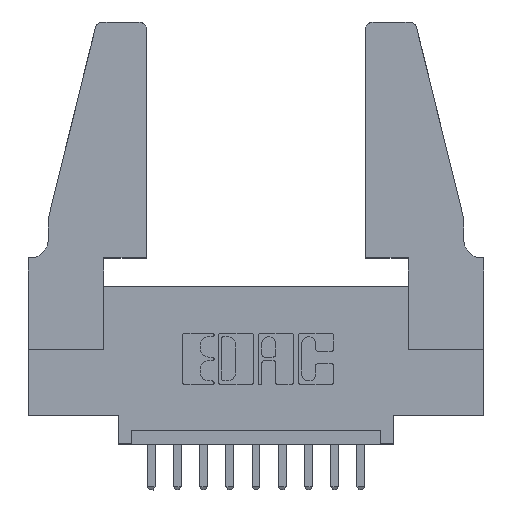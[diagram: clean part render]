
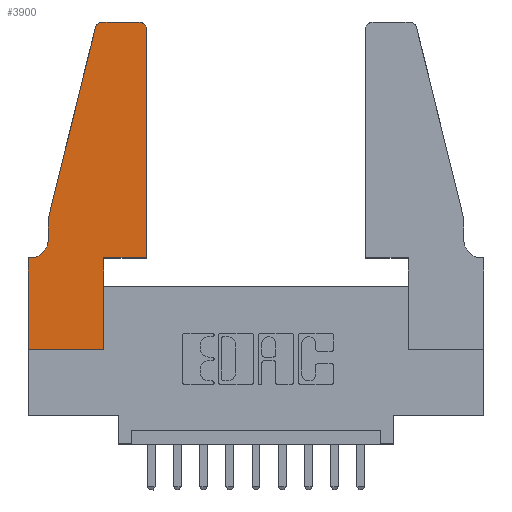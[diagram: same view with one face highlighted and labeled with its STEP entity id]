
A CAD part, top view. The second image highlights one B-rep face of the part: STEP entity #3900.
In plain terms, the highlighted planar face has unit normal (0, 0, 1).
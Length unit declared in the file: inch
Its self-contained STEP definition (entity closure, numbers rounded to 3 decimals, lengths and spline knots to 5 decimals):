
#124 = DIRECTION ( 'NONE',  ( 1., 0., 0. ) ) ;
#148 = DIRECTION ( 'NONE',  ( 1., 0., 0. ) ) ;
#385 = EDGE_CURVE ( 'NONE', #1958, #7361, #8464, .T. ) ;
#652 = ORIENTED_EDGE ( 'NONE', *, *, #8223, .T. ) ;
#665 = ORIENTED_EDGE ( 'NONE', *, *, #12325, .T. ) ;
#725 = EDGE_CURVE ( 'NONE', #7361, #761, #2554, .T. ) ;
#761 = VERTEX_POINT ( 'NONE', #7564 ) ;
#826 = VERTEX_POINT ( 'NONE', #6489 ) ;
#1032 = LINE ( 'NONE', #9588, #8779 ) ;
#1060 = DIRECTION ( 'NONE',  ( 0., 0., 1. ) ) ;
#1082 = LINE ( 'NONE', #9185, #13083 ) ;
#1126 = EDGE_CURVE ( 'NONE', #11859, #2603, #1032, .T. ) ;
#1560 = AXIS2_PLACEMENT_3D ( 'NONE', #7431, #5410, #124 ) ;
#1623 = AXIS2_PLACEMENT_3D ( 'NONE', #11370, #8103, #9340 ) ;
#1958 = VERTEX_POINT ( 'NONE', #4725 ) ;
#2005 = DIRECTION ( 'NONE',  ( 0., 1., 0. ) ) ;
#2279 = FACE_OUTER_BOUND ( 'NONE', #11975, .T. ) ;
#2554 = CIRCLE ( 'NONE', #6202, 0.03 ) ;
#2603 = VERTEX_POINT ( 'NONE', #5949 ) ;
#2647 = CARTESIAN_POINT ( 'NONE',  ( 0.0755, 0.5, 0.37 ) ) ;
#2733 = CARTESIAN_POINT ( 'NONE',  ( 0.4505, 0.35, 0.37 ) ) ;
#2842 = ORIENTED_EDGE ( 'NONE', *, *, #7380, .T. ) ;
#2963 = DIRECTION ( 'NONE',  ( 1., 0., 0. ) ) ;
#3013 = CARTESIAN_POINT ( 'NONE',  ( 0.2865, 0.35, 0.37 ) ) ;
#3455 = CIRCLE ( 'NONE', #1623, 0.07 ) ;
#3594 = EDGE_CURVE ( 'NONE', #10299, #4661, #10351, .T. ) ;
#3641 = CARTESIAN_POINT ( 'NONE',  ( 0., 0., 0.37 ) ) ;
#3900 = ADVANCED_FACE ( 'NONE', ( #2279 ), #11563, .T. ) ;
#4121 = CARTESIAN_POINT ( 'NONE',  ( 0.4505, 0.35, 0.37 ) ) ;
#4207 = CARTESIAN_POINT ( 'NONE',  ( 0.284, 1.22, 0.37 ) ) ;
#4279 = LINE ( 'NONE', #2647, #9853 ) ;
#4661 = VERTEX_POINT ( 'NONE', #11516 ) ;
#4725 = CARTESIAN_POINT ( 'NONE',  ( 0.4205, 1.25, 0.37 ) ) ;
#4775 = VECTOR ( 'NONE', #7015, 39.37008 ) ;
#4886 = CARTESIAN_POINT ( 'NONE',  ( 0.0755, 0.5, 0.37 ) ) ;
#5058 = ORIENTED_EDGE ( 'NONE', *, *, #11753, .T. ) ;
#5268 = DIRECTION ( 'NONE',  ( 1., 0., 0. ) ) ;
#5410 = DIRECTION ( 'NONE',  ( 0., 0., 1. ) ) ;
#5949 = CARTESIAN_POINT ( 'NONE',  ( 0.2865, 0., 0.37 ) ) ;
#6174 = DIRECTION ( 'NONE',  ( -1., 0., 0. ) ) ;
#6202 = AXIS2_PLACEMENT_3D ( 'NONE', #4207, #6250, #5268 ) ;
#6250 = DIRECTION ( 'NONE',  ( 0., 0., 1. ) ) ;
#6489 = CARTESIAN_POINT ( 'NONE',  ( 0.4505, 0.35, 0.37 ) ) ;
#6818 = DIRECTION ( 'NONE',  ( -1., 0., 0. ) ) ;
#6920 = VECTOR ( 'NONE', #2005, 39.37008 ) ;
#7015 = DIRECTION ( 'NONE',  ( 0., -1., 0. ) ) ;
#7305 = VERTEX_POINT ( 'NONE', #8635 ) ;
#7361 = VERTEX_POINT ( 'NONE', #10802 ) ;
#7380 = EDGE_CURVE ( 'NONE', #7717, #826, #9242, .T. ) ;
#7382 = ORIENTED_EDGE ( 'NONE', *, *, #8162, .T. ) ;
#7387 = CIRCLE ( 'NONE', #1560, 0.03 ) ;
#7388 = CARTESIAN_POINT ( 'NONE',  ( 0.0055, 0.35, 0.37 ) ) ;
#7431 = CARTESIAN_POINT ( 'NONE',  ( 0.4205, 1.22, 0.37 ) ) ;
#7536 = CARTESIAN_POINT ( 'NONE',  ( 0., 0., 0.37 ) ) ;
#7564 = CARTESIAN_POINT ( 'NONE',  ( 0.25487, 1.22718, 0.37 ) ) ;
#7604 = ORIENTED_EDGE ( 'NONE', *, *, #1126, .T. ) ;
#7717 = VERTEX_POINT ( 'NONE', #13519 ) ;
#7998 = VERTEX_POINT ( 'NONE', #8800 ) ;
#8103 = DIRECTION ( 'NONE',  ( 0., 0., -1. ) ) ;
#8162 = EDGE_CURVE ( 'NONE', #761, #10299, #4279, .T. ) ;
#8223 = EDGE_CURVE ( 'NONE', #4661, #13224, #3455, .T. ) ;
#8399 = ORIENTED_EDGE ( 'NONE', *, *, #385, .T. ) ;
#8464 = LINE ( 'NONE', #13151, #10937 ) ;
#8635 = CARTESIAN_POINT ( 'NONE',  ( 0.4505, 1.22, 0.37 ) ) ;
#8779 = VECTOR ( 'NONE', #148, 39.37008 ) ;
#8800 = CARTESIAN_POINT ( 'NONE',  ( 0., 0.35, 0.37 ) ) ;
#8975 = VECTOR ( 'NONE', #12380, 39.37008 ) ;
#9185 = CARTESIAN_POINT ( 'NONE',  ( 0.0755, 0.35, 0.37 ) ) ;
#9242 = LINE ( 'NONE', #2733, #12825 ) ;
#9310 = ORIENTED_EDGE ( 'NONE', *, *, #11044, .T. ) ;
#9318 = ORIENTED_EDGE ( 'NONE', *, *, #12968, .T. ) ;
#9340 = DIRECTION ( 'NONE',  ( -1., 0., 0. ) ) ;
#9588 = CARTESIAN_POINT ( 'NONE',  ( 0., 0., 0.37 ) ) ;
#9853 = VECTOR ( 'NONE', #12178, 39.37008 ) ;
#10015 = VECTOR ( 'NONE', #10650, 39.37008 ) ;
#10045 = CARTESIAN_POINT ( 'NONE',  ( 0.0755, 0.5, 0.37 ) ) ;
#10078 = DIRECTION ( 'NONE',  ( 1., 0., 0. ) ) ;
#10079 = ORIENTED_EDGE ( 'NONE', *, *, #3594, .T. ) ;
#10299 = VERTEX_POINT ( 'NONE', #10045 ) ;
#10351 = LINE ( 'NONE', #4886, #4775 ) ;
#10650 = DIRECTION ( 'NONE',  ( 0., -1., 0. ) ) ;
#10677 = LINE ( 'NONE', #7536, #10015 ) ;
#10802 = CARTESIAN_POINT ( 'NONE',  ( 0.284, 1.25, 0.37 ) ) ;
#10937 = VECTOR ( 'NONE', #6818, 39.37008 ) ;
#11044 = EDGE_CURVE ( 'NONE', #2603, #7717, #13219, .T. ) ;
#11370 = CARTESIAN_POINT ( 'NONE',  ( 0.0055, 0.42, 0.37 ) ) ;
#11516 = CARTESIAN_POINT ( 'NONE',  ( 0.0755, 0.42, 0.37 ) ) ;
#11563 = PLANE ( 'NONE',  #12626 ) ;
#11734 = ORIENTED_EDGE ( 'NONE', *, *, #725, .T. ) ;
#11753 = EDGE_CURVE ( 'NONE', #7998, #11859, #10677, .T. ) ;
#11859 = VERTEX_POINT ( 'NONE', #3641 ) ;
#11975 = EDGE_LOOP ( 'NONE', ( #8399, #11734, #7382, #10079, #652, #9318, #5058, #7604, #9310, #2842, #665, #13222 ) ) ;
#12178 = DIRECTION ( 'NONE',  ( -0.239, -0.971, 0. ) ) ;
#12325 = EDGE_CURVE ( 'NONE', #826, #7305, #12933, .T. ) ;
#12357 = EDGE_CURVE ( 'NONE', #7305, #1958, #7387, .T. ) ;
#12380 = DIRECTION ( 'NONE',  ( 0., 1., 0. ) ) ;
#12626 = AXIS2_PLACEMENT_3D ( 'NONE', #13645, #1060, #2963 ) ;
#12825 = VECTOR ( 'NONE', #10078, 39.37008 ) ;
#12933 = LINE ( 'NONE', #4121, #6920 ) ;
#12968 = EDGE_CURVE ( 'NONE', #13224, #7998, #1082, .T. ) ;
#13083 = VECTOR ( 'NONE', #6174, 39.37008 ) ;
#13151 = CARTESIAN_POINT ( 'NONE',  ( 0.2605, 1.25, 0.37 ) ) ;
#13219 = LINE ( 'NONE', #3013, #8975 ) ;
#13222 = ORIENTED_EDGE ( 'NONE', *, *, #12357, .T. ) ;
#13224 = VERTEX_POINT ( 'NONE', #7388 ) ;
#13519 = CARTESIAN_POINT ( 'NONE',  ( 0.2865, 0.35, 0.37 ) ) ;
#13645 = CARTESIAN_POINT ( 'NONE',  ( 0., 0.35, 0.37 ) ) ;
